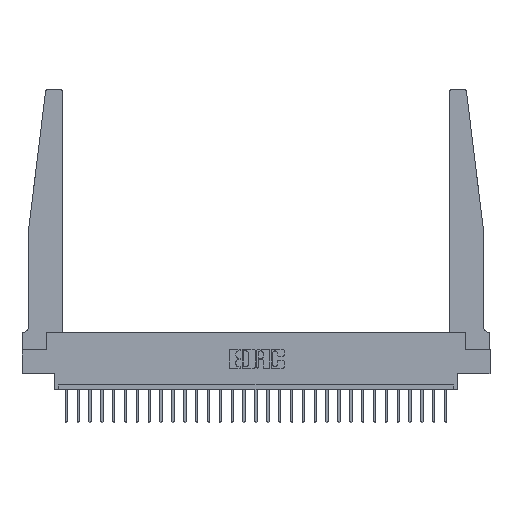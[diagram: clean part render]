
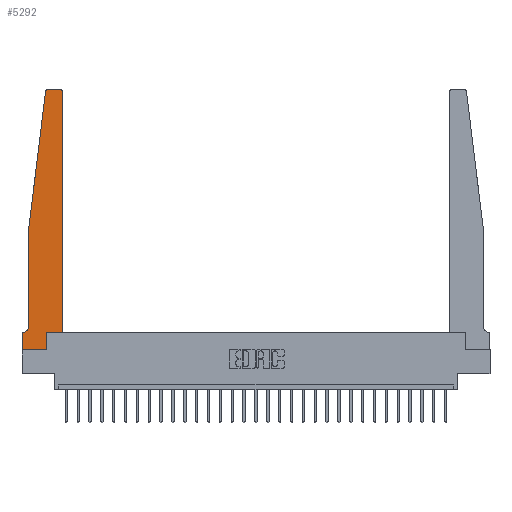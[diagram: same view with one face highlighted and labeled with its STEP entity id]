
A CAD part, top view. The second image highlights one B-rep face of the part: STEP entity #5292.
In plain terms, the highlighted planar face has unit normal (0, 0, 1).
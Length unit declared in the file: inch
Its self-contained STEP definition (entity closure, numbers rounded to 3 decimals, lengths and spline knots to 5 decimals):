
#522 = LINE ( 'NONE', #9252, #6988 ) ;
#807 = EDGE_CURVE ( 'NONE', #25887, #20410, #6187, .T. ) ;
#901 = CARTESIAN_POINT ( 'NONE',  ( 0.27653, 2.72, 0.37 ) ) ;
#1031 = DIRECTION ( 'NONE',  ( 1., 0., 0. ) ) ;
#1299 = EDGE_CURVE ( 'NONE', #13350, #6682, #4755, .T. ) ;
#1739 = ORIENTED_EDGE ( 'NONE', *, *, #807, .T. ) ;
#1976 = EDGE_LOOP ( 'NONE', ( #12918, #8793, #24136, #3570, #1739, #7550, #23335, #15604, #23205, #11113, #18699, #8444 ) ) ;
#2062 = CARTESIAN_POINT ( 'NONE',  ( 0.2605, 0., 0.37 ) ) ;
#2317 = EDGE_CURVE ( 'NONE', #26001, #13350, #25472, .T. ) ;
#2794 = LINE ( 'NONE', #4588, #10645 ) ;
#2932 = CARTESIAN_POINT ( 'NONE',  ( 0.015, 0.2375, 0.37 ) ) ;
#3109 = DIRECTION ( 'NONE',  ( 0., -1., 0. ) ) ;
#3146 = CARTESIAN_POINT ( 'NONE',  ( 0.065, 1.25, 0.37 ) ) ;
#3570 = ORIENTED_EDGE ( 'NONE', *, *, #12975, .T. ) ;
#3937 = AXIS2_PLACEMENT_3D ( 'NONE', #26500, #7763, #26639 ) ;
#4192 = DIRECTION ( 'NONE',  ( 1., 0., 0. ) ) ;
#4588 = CARTESIAN_POINT ( 'NONE',  ( 0., 0., 0.37 ) ) ;
#4755 = LINE ( 'NONE', #13050, #10941 ) ;
#4886 = DIRECTION ( 'NONE',  ( 0., 1., 0. ) ) ;
#5134 = CARTESIAN_POINT ( 'NONE',  ( 0., 0.1875, 0.37 ) ) ;
#5174 = EDGE_CURVE ( 'NONE', #6682, #22158, #16570, .T. ) ;
#5292 = ADVANCED_FACE ( 'NONE', ( #20210 ), #9781, .T. ) ;
#5718 = CARTESIAN_POINT ( 'NONE',  ( 0.395, 2.72, 0.37 ) ) ;
#6110 = VERTEX_POINT ( 'NONE', #18488 ) ;
#6187 = CIRCLE ( 'NONE', #24047, 0.05 ) ;
#6682 = VERTEX_POINT ( 'NONE', #12337 ) ;
#6836 = EDGE_CURVE ( 'NONE', #7901, #20302, #2794, .T. ) ;
#6844 = CARTESIAN_POINT ( 'NONE',  ( 0.065, 0.1875, 0.37 ) ) ;
#6988 = VECTOR ( 'NONE', #3109, 39.37008 ) ;
#7550 = ORIENTED_EDGE ( 'NONE', *, *, #25228, .T. ) ;
#7583 = EDGE_CURVE ( 'NONE', #15074, #7901, #522, .T. ) ;
#7625 = CARTESIAN_POINT ( 'NONE',  ( 0.425, 0.18, 0.37 ) ) ;
#7763 = DIRECTION ( 'NONE',  ( 0., 0., 1. ) ) ;
#7901 = VERTEX_POINT ( 'NONE', #16485 ) ;
#8007 = CARTESIAN_POINT ( 'NONE',  ( 0.065, 0.2375, 0.37 ) ) ;
#8444 = ORIENTED_EDGE ( 'NONE', *, *, #5174, .T. ) ;
#8613 = DIRECTION ( 'NONE',  ( -1., 0., 0. ) ) ;
#8793 = ORIENTED_EDGE ( 'NONE', *, *, #25744, .T. ) ;
#9252 = CARTESIAN_POINT ( 'NONE',  ( 0., 0., 0.37 ) ) ;
#9781 = PLANE ( 'NONE',  #3937 ) ;
#10168 = CARTESIAN_POINT ( 'NONE',  ( 0.395, 2.75, 0.37 ) ) ;
#10215 = DIRECTION ( 'NONE',  ( 0., -1., 0. ) ) ;
#10645 = VECTOR ( 'NONE', #21294, 39.37008 ) ;
#10766 = LINE ( 'NONE', #6844, #25699 ) ;
#10941 = VECTOR ( 'NONE', #4886, 39.37008 ) ;
#11113 = ORIENTED_EDGE ( 'NONE', *, *, #2317, .T. ) ;
#11684 = DIRECTION ( 'NONE',  ( 1., 0., 0. ) ) ;
#11689 = CARTESIAN_POINT ( 'NONE',  ( 0.015, 0.1875, 0.37 ) ) ;
#12337 = CARTESIAN_POINT ( 'NONE',  ( 0.425, 2.72, 0.37 ) ) ;
#12597 = AXIS2_PLACEMENT_3D ( 'NONE', #5718, #26779, #11684 ) ;
#12879 = DIRECTION ( 'NONE',  ( 0., 0., -1. ) ) ;
#12918 = ORIENTED_EDGE ( 'NONE', *, *, #26109, .T. ) ;
#12975 = EDGE_CURVE ( 'NONE', #14031, #25887, #18455, .T. ) ;
#13050 = CARTESIAN_POINT ( 'NONE',  ( 0.425, 0.18, 0.37 ) ) ;
#13350 = VERTEX_POINT ( 'NONE', #7625 ) ;
#14031 = VERTEX_POINT ( 'NONE', #3146 ) ;
#14038 = LINE ( 'NONE', #18467, #21307 ) ;
#14110 = CARTESIAN_POINT ( 'NONE',  ( 0.2605, 0.18, 0.37 ) ) ;
#14225 = EDGE_CURVE ( 'NONE', #20302, #26001, #16663, .T. ) ;
#14818 = CARTESIAN_POINT ( 'NONE',  ( 0.25, 2.75, 0.37 ) ) ;
#15074 = VERTEX_POINT ( 'NONE', #5134 ) ;
#15519 = DIRECTION ( 'NONE',  ( 0., 0., 1. ) ) ;
#15604 = ORIENTED_EDGE ( 'NONE', *, *, #6836, .T. ) ;
#16485 = CARTESIAN_POINT ( 'NONE',  ( 0., 0., 0.37 ) ) ;
#16570 = CIRCLE ( 'NONE', #12597, 0.03 ) ;
#16663 = LINE ( 'NONE', #19269, #22539 ) ;
#17180 = VERTEX_POINT ( 'NONE', #18071 ) ;
#18071 = CARTESIAN_POINT ( 'NONE',  ( 0.24675, 2.72367, 0.37 ) ) ;
#18455 = LINE ( 'NONE', #26673, #22544 ) ;
#18467 = CARTESIAN_POINT ( 'NONE',  ( 0.065, 1.25, 0.37 ) ) ;
#18488 = CARTESIAN_POINT ( 'NONE',  ( 0.27653, 2.75, 0.37 ) ) ;
#18699 = ORIENTED_EDGE ( 'NONE', *, *, #1299, .T. ) ;
#19143 = EDGE_CURVE ( 'NONE', #17180, #14031, #14038, .T. ) ;
#19269 = CARTESIAN_POINT ( 'NONE',  ( 0.2605, 0.18, 0.37 ) ) ;
#19959 = VECTOR ( 'NONE', #4192, 39.37008 ) ;
#20210 = FACE_OUTER_BOUND ( 'NONE', #1976, .T. ) ;
#20302 = VERTEX_POINT ( 'NONE', #2062 ) ;
#20410 = VERTEX_POINT ( 'NONE', #11689 ) ;
#20952 = AXIS2_PLACEMENT_3D ( 'NONE', #901, #15519, #1031 ) ;
#21284 = DIRECTION ( 'NONE',  ( -1., 0., 0. ) ) ;
#21294 = DIRECTION ( 'NONE',  ( 1., 0., 0. ) ) ;
#21299 = DIRECTION ( 'NONE',  ( -1., 0., 0. ) ) ;
#21307 = VECTOR ( 'NONE', #22712, 39.37008 ) ;
#22158 = VERTEX_POINT ( 'NONE', #10168 ) ;
#22272 = VECTOR ( 'NONE', #21284, 39.37008 ) ;
#22539 = VECTOR ( 'NONE', #25029, 39.37008 ) ;
#22544 = VECTOR ( 'NONE', #10215, 39.37008 ) ;
#22712 = DIRECTION ( 'NONE',  ( -0.122, -0.992, 0. ) ) ;
#23187 = LINE ( 'NONE', #14818, #22272 ) ;
#23205 = ORIENTED_EDGE ( 'NONE', *, *, #14225, .T. ) ;
#23335 = ORIENTED_EDGE ( 'NONE', *, *, #7583, .T. ) ;
#24047 = AXIS2_PLACEMENT_3D ( 'NONE', #2932, #12879, #21299 ) ;
#24136 = ORIENTED_EDGE ( 'NONE', *, *, #19143, .T. ) ;
#24977 = CARTESIAN_POINT ( 'NONE',  ( 0.425, 0.18, 0.37 ) ) ;
#25029 = DIRECTION ( 'NONE',  ( 0., 1., 0. ) ) ;
#25228 = EDGE_CURVE ( 'NONE', #20410, #15074, #10766, .T. ) ;
#25284 = CIRCLE ( 'NONE', #20952, 0.03 ) ;
#25472 = LINE ( 'NONE', #24977, #19959 ) ;
#25699 = VECTOR ( 'NONE', #8613, 39.37008 ) ;
#25744 = EDGE_CURVE ( 'NONE', #6110, #17180, #25284, .T. ) ;
#25887 = VERTEX_POINT ( 'NONE', #8007 ) ;
#26001 = VERTEX_POINT ( 'NONE', #14110 ) ;
#26109 = EDGE_CURVE ( 'NONE', #22158, #6110, #23187, .T. ) ;
#26500 = CARTESIAN_POINT ( 'NONE',  ( 0., 0.1875, 0.37 ) ) ;
#26639 = DIRECTION ( 'NONE',  ( 1., 0., 0. ) ) ;
#26673 = CARTESIAN_POINT ( 'NONE',  ( 0.065, 1.25, 0.37 ) ) ;
#26779 = DIRECTION ( 'NONE',  ( 0., 0., 1. ) ) ;
